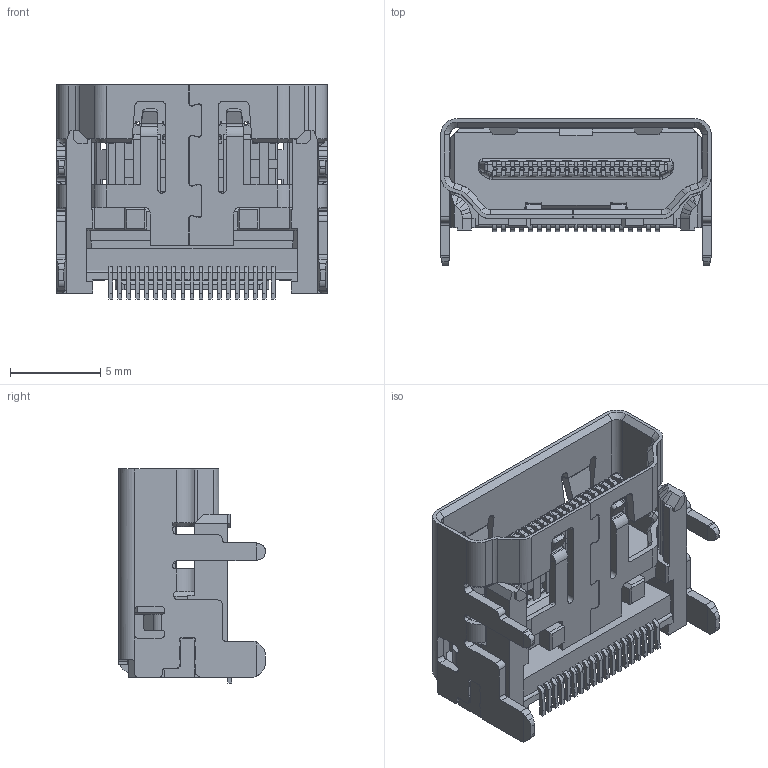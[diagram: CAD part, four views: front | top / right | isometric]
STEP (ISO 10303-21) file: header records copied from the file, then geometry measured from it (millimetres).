
FILE_DESCRIPTION (( 'STEP AP214' ), '1' );
FILE_NAME ('694A619-164-011.STEP', '2021-01-13T13:22:44', ( '' ), ( '' ), 'SwSTEP 2.0', 'SolidWorks 2020', '' );
FILE_SCHEMA (( 'AUTOMOTIVE_DESIGN' ));
Length unit declared in the file: millimetre
Products named in the file (3): Insulator 694A619-X64-011; 694A619-164-011; Shell 694A619-X64-011
Assembly tree (2 placements, depth 2):
  694A619-164-011
    Insulator 694A619-X64-011
    Shell 694A619-X64-011
Bounding box: 15 x 8.13 x 11.87 mm (x, y, z)
Volume: 461.8 mm3; surface area: 1590.3 mm2
Topology: 2 solids, 2 shells, 2032 faces, 5947 edges, 3881 vertices
Faces by surface type: plane 1473, cylinder 480, bspline 51, cone 27, torus 1
Entity records: 75369 total; most frequent: CARTESIAN_POINT 18590, ORIENTED_EDGE 11890, DIRECTION 9006, EDGE_CURVE 5945, VECTOR 4156, LINE 4156, VERTEX_POINT 3881, AXIS2_PLACEMENT_3D 2425
